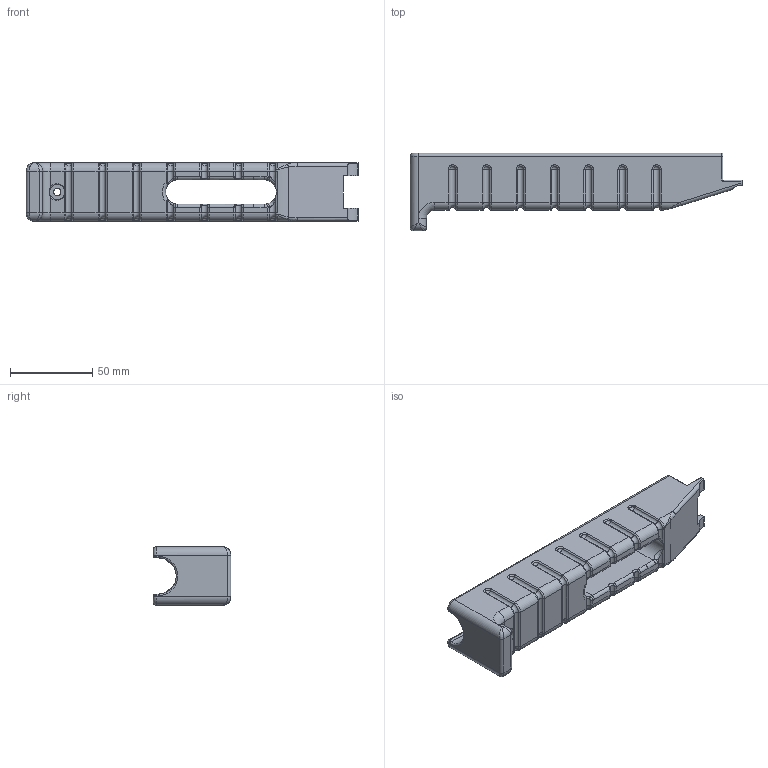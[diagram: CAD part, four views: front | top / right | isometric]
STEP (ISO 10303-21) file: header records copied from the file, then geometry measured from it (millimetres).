
FILE_DESCRIPTION(/* description */ (''),/* implementation_level */ '2;1');
FILE_NAME(/* name */ 'Hatfield Handguard.step',/* time_stamp */ '2021-05-20T08:25:20-06:00',/* author */ (''),/* organization */ (''),/* preprocessor_version */ 'ST-DEVELOPER v18.1',/* originating_system */ 'Autodesk Translation Framework v10.6.0.1341',/* authorisation */ '');
FILE_SCHEMA (('AUTOMOTIVE_DESIGN { 1 0 10303 214 3 1 1 }'));
Length unit declared in the file: millimetre
Products named in the file (1): Hatfield Projects
Bounding box: 201.98 x 47.29 x 35.5 mm (x, y, z)
Volume: 143726.9 mm3; surface area: 34541.1 mm2
Topology: 1 solids, 1 shells, 310 faces, 709 edges, 395 vertices
Faces by surface type: cylinder 138, torus 76, bspline 41, plane 40, sphere 14, cone 1
Full cylindrical faces by diameter (mm): 4.5 x1, 9.5 x1, 11 x1
Entity records: 10497 total; most frequent: CARTESIAN_POINT 3606, DIRECTION 1520, ORIENTED_EDGE 1406, EDGE_CURVE 703, AXIS2_PLACEMENT_3D 633, VERTEX_POINT 395, CIRCLE 339, EDGE_LOOP 314
